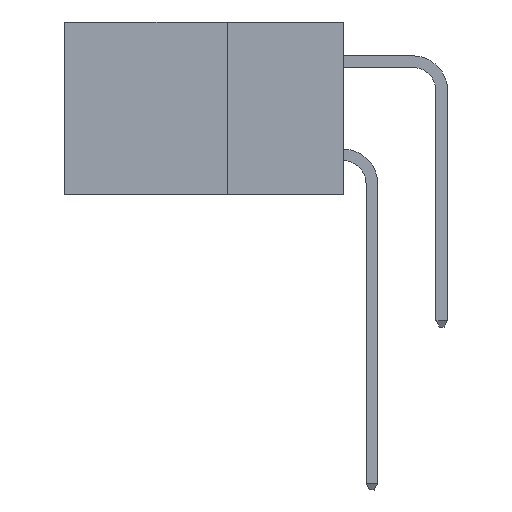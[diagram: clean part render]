
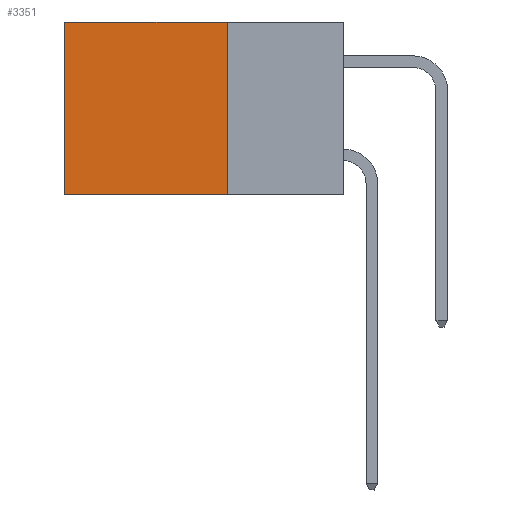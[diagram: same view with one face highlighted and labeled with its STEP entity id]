
A CAD part, left-side view. The second image highlights one B-rep face of the part: STEP entity #3351.
In plain terms, the highlighted planar face has unit normal (-1, 0, 0).
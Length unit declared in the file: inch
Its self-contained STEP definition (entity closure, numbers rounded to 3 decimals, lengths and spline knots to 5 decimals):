
#50 = EDGE_CURVE ( 'NONE', #4900, #14485, #10406, .T. ) ;
#177 = DIRECTION ( 'NONE',  ( 0., 1., 0. ) ) ;
#243 = CARTESIAN_POINT ( 'NONE',  ( 0.298, 0.25, 0. ) ) ;
#1008 = CARTESIAN_POINT ( 'NONE',  ( 0.298, 0.25, -0.37 ) ) ;
#1193 = CARTESIAN_POINT ( 'NONE',  ( 0.298, 0.25, 0. ) ) ;
#1961 = CARTESIAN_POINT ( 'NONE',  ( 0.298, 0.6, 0. ) ) ;
#2402 = ORIENTED_EDGE ( 'NONE', *, *, #9649, .F. ) ;
#3077 = EDGE_CURVE ( 'NONE', #14485, #14416, #16890, .T. ) ;
#3351 = ADVANCED_FACE ( 'NONE', ( #28290 ), #26288, .F. ) ;
#4089 = DIRECTION ( 'NONE',  ( 0., 1., 0. ) ) ;
#4883 = VERTEX_POINT ( 'NONE', #9846 ) ;
#4900 = VERTEX_POINT ( 'NONE', #13539 ) ;
#4965 = CARTESIAN_POINT ( 'NONE',  ( 0.298, 0.6, 0. ) ) ;
#7627 = EDGE_CURVE ( 'NONE', #4883, #14416, #30630, .T. ) ;
#9566 = ORIENTED_EDGE ( 'NONE', *, *, #7627, .F. ) ;
#9649 = EDGE_CURVE ( 'NONE', #4900, #4883, #10066, .T. ) ;
#9846 = CARTESIAN_POINT ( 'NONE',  ( 0.298, 0.25, -0.37 ) ) ;
#10066 = LINE ( 'NONE', #21350, #29355 ) ;
#10406 = LINE ( 'NONE', #1193, #31222 ) ;
#10597 = VECTOR ( 'NONE', #177, 39.37008 ) ;
#13539 = CARTESIAN_POINT ( 'NONE',  ( 0.298, 0.25, 0. ) ) ;
#14416 = VERTEX_POINT ( 'NONE', #16811 ) ;
#14485 = VERTEX_POINT ( 'NONE', #1961 ) ;
#16811 = CARTESIAN_POINT ( 'NONE',  ( 0.298, 0.6, -0.37 ) ) ;
#16890 = LINE ( 'NONE', #4965, #17679 ) ;
#17679 = VECTOR ( 'NONE', #23000, 39.37008 ) ;
#19491 = ORIENTED_EDGE ( 'NONE', *, *, #3077, .T. ) ;
#21350 = CARTESIAN_POINT ( 'NONE',  ( 0.298, 0.25, 0. ) ) ;
#23000 = DIRECTION ( 'NONE',  ( 0., 0., -1. ) ) ;
#23018 = DIRECTION ( 'NONE',  ( 0., 0., -1. ) ) ;
#23220 = DIRECTION ( 'NONE',  ( 1., 0., 0. ) ) ;
#24019 = ORIENTED_EDGE ( 'NONE', *, *, #50, .T. ) ;
#24761 = AXIS2_PLACEMENT_3D ( 'NONE', #243, #23220, #23018 ) ;
#25046 = EDGE_LOOP ( 'NONE', ( #19491, #9566, #2402, #24019 ) ) ;
#26288 = PLANE ( 'NONE',  #24761 ) ;
#28290 = FACE_OUTER_BOUND ( 'NONE', #25046, .T. ) ;
#28933 = DIRECTION ( 'NONE',  ( 0., 0., -1. ) ) ;
#29355 = VECTOR ( 'NONE', #28933, 39.37008 ) ;
#30630 = LINE ( 'NONE', #1008, #10597 ) ;
#31222 = VECTOR ( 'NONE', #4089, 39.37008 ) ;
